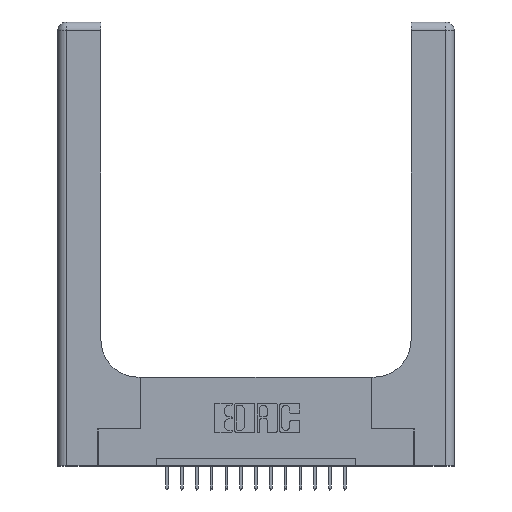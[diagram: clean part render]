
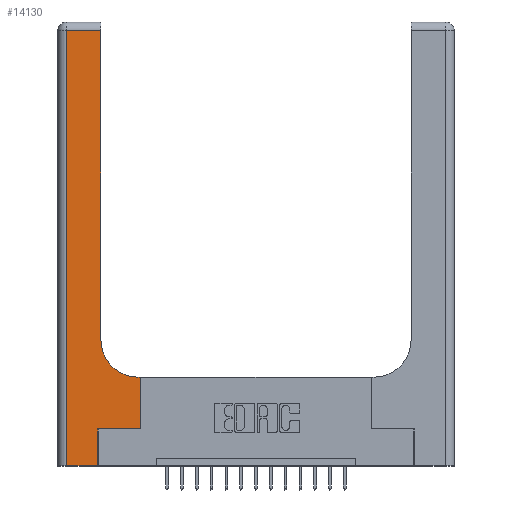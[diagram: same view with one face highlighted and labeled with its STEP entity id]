
A CAD part, top view. The second image highlights one B-rep face of the part: STEP entity #14130.
In plain terms, the highlighted planar face has unit normal (0, 0, 1).
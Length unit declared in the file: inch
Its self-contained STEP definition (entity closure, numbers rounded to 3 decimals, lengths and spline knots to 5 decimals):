
#91 = CARTESIAN_POINT ( 'NONE',  ( 0.2915, 3., 0.37 ) ) ;
#858 = DIRECTION ( 'NONE',  ( 0., 1., 0. ) ) ;
#987 = VECTOR ( 'NONE', #13800, 39.37008 ) ;
#1414 = ORIENTED_EDGE ( 'NONE', *, *, #1818, .T. ) ;
#1717 = CARTESIAN_POINT ( 'NONE',  ( 0.2915, 0.6, 0.37 ) ) ;
#1818 = EDGE_CURVE ( 'NONE', #18265, #15217, #3611, .T. ) ;
#1908 = CARTESIAN_POINT ( 'NONE',  ( 0.06, 0., 0.37 ) ) ;
#2153 = LINE ( 'NONE', #5786, #16778 ) ;
#2196 = ORIENTED_EDGE ( 'NONE', *, *, #6214, .T. ) ;
#2522 = DIRECTION ( 'NONE',  ( 0., 0., -1. ) ) ;
#2661 = DIRECTION ( 'NONE',  ( 1., 0., 0. ) ) ;
#2666 = ORIENTED_EDGE ( 'NONE', *, *, #7473, .T. ) ;
#2772 = VERTEX_POINT ( 'NONE', #1908 ) ;
#2823 = VECTOR ( 'NONE', #11166, 39.37008 ) ;
#3020 = DIRECTION ( 'NONE',  ( 0., 1., 0. ) ) ;
#3329 = VECTOR ( 'NONE', #18202, 39.37008 ) ;
#3611 = CIRCLE ( 'NONE', #15936, 0.25 ) ;
#3687 = ORIENTED_EDGE ( 'NONE', *, *, #12773, .T. ) ;
#4077 = CARTESIAN_POINT ( 'NONE',  ( 0.5415, 0.85, 0.37 ) ) ;
#4161 = EDGE_CURVE ( 'NONE', #15096, #11224, #2153, .T. ) ;
#4436 = ORIENTED_EDGE ( 'NONE', *, *, #16899, .T. ) ;
#4519 = VERTEX_POINT ( 'NONE', #13186 ) ;
#5191 = ORIENTED_EDGE ( 'NONE', *, *, #16734, .T. ) ;
#5257 = CARTESIAN_POINT ( 'NONE',  ( 0.2915, 0.85, 0.37 ) ) ;
#5313 = DIRECTION ( 'NONE',  ( 0., 1., 0. ) ) ;
#5616 = DIRECTION ( 'NONE',  ( -1., 0., 0. ) ) ;
#5687 = CARTESIAN_POINT ( 'NONE',  ( 0., 2.94, 0.37 ) ) ;
#5735 = VECTOR ( 'NONE', #3020, 39.37008 ) ;
#5786 = CARTESIAN_POINT ( 'NONE',  ( 0.5585, 0.25, 0.37 ) ) ;
#6214 = EDGE_CURVE ( 'NONE', #4519, #2772, #14758, .T. ) ;
#6222 = CARTESIAN_POINT ( 'NONE',  ( 0.5585, 0.25, 0.37 ) ) ;
#6415 = VECTOR ( 'NONE', #858, 39.37008 ) ;
#7250 = CARTESIAN_POINT ( 'NONE',  ( 0.5585, 0.6, 0.37 ) ) ;
#7461 = VECTOR ( 'NONE', #5616, 39.37008 ) ;
#7473 = EDGE_CURVE ( 'NONE', #11224, #18265, #11968, .T. ) ;
#7494 = EDGE_LOOP ( 'NONE', ( #3687, #7683, #2196, #4436, #8597, #5191, #10082, #2666, #1414 ) ) ;
#7683 = ORIENTED_EDGE ( 'NONE', *, *, #18147, .T. ) ;
#8170 = PLANE ( 'NONE',  #11395 ) ;
#8458 = VERTEX_POINT ( 'NONE', #8619 ) ;
#8523 = DIRECTION ( 'NONE',  ( 1., 0., 0. ) ) ;
#8597 = ORIENTED_EDGE ( 'NONE', *, *, #13118, .T. ) ;
#8619 = CARTESIAN_POINT ( 'NONE',  ( 0.2915, 2.94, 0.37 ) ) ;
#9448 = CARTESIAN_POINT ( 'NONE',  ( 0.269, 0.25, 0.37 ) ) ;
#9609 = LINE ( 'NONE', #91, #5735 ) ;
#10082 = ORIENTED_EDGE ( 'NONE', *, *, #4161, .T. ) ;
#10148 = LINE ( 'NONE', #11226, #11975 ) ;
#10279 = CARTESIAN_POINT ( 'NONE',  ( 0.5415, 0.6, 0.37 ) ) ;
#10475 = FACE_OUTER_BOUND ( 'NONE', #7494, .T. ) ;
#11166 = DIRECTION ( 'NONE',  ( 1., 0., 0. ) ) ;
#11224 = VERTEX_POINT ( 'NONE', #7250 ) ;
#11226 = CARTESIAN_POINT ( 'NONE',  ( 0., 0., 0.37 ) ) ;
#11395 = AXIS2_PLACEMENT_3D ( 'NONE', #12584, #14064, #15510 ) ;
#11899 = VERTEX_POINT ( 'NONE', #15185 ) ;
#11968 = LINE ( 'NONE', #1717, #987 ) ;
#11975 = VECTOR ( 'NONE', #8523, 39.37008 ) ;
#12584 = CARTESIAN_POINT ( 'NONE',  ( 0., 3., 0.37 ) ) ;
#12773 = EDGE_CURVE ( 'NONE', #15217, #8458, #9609, .T. ) ;
#13118 = EDGE_CURVE ( 'NONE', #11899, #17457, #13498, .T. ) ;
#13186 = CARTESIAN_POINT ( 'NONE',  ( 0.06, 2.94, 0.37 ) ) ;
#13498 = LINE ( 'NONE', #18502, #6415 ) ;
#13800 = DIRECTION ( 'NONE',  ( -1., 0., 0. ) ) ;
#14064 = DIRECTION ( 'NONE',  ( 0., 0., -1. ) ) ;
#14130 = ADVANCED_FACE ( 'NONE', ( #10475 ), #8170, .F. ) ;
#14758 = LINE ( 'NONE', #16720, #3329 ) ;
#15096 = VERTEX_POINT ( 'NONE', #6222 ) ;
#15185 = CARTESIAN_POINT ( 'NONE',  ( 0.269, 0., 0.37 ) ) ;
#15217 = VERTEX_POINT ( 'NONE', #5257 ) ;
#15225 = LINE ( 'NONE', #5687, #7461 ) ;
#15510 = DIRECTION ( 'NONE',  ( -1., 0., 0. ) ) ;
#15852 = CARTESIAN_POINT ( 'NONE',  ( 0.269, 0.25, 0.37 ) ) ;
#15936 = AXIS2_PLACEMENT_3D ( 'NONE', #4077, #2522, #2661 ) ;
#16720 = CARTESIAN_POINT ( 'NONE',  ( 0.06, 3., 0.37 ) ) ;
#16734 = EDGE_CURVE ( 'NONE', #17457, #15096, #17012, .T. ) ;
#16778 = VECTOR ( 'NONE', #5313, 39.37008 ) ;
#16899 = EDGE_CURVE ( 'NONE', #2772, #11899, #10148, .T. ) ;
#17012 = LINE ( 'NONE', #9448, #2823 ) ;
#17457 = VERTEX_POINT ( 'NONE', #15852 ) ;
#18147 = EDGE_CURVE ( 'NONE', #8458, #4519, #15225, .T. ) ;
#18202 = DIRECTION ( 'NONE',  ( 0., -1., 0. ) ) ;
#18265 = VERTEX_POINT ( 'NONE', #10279 ) ;
#18502 = CARTESIAN_POINT ( 'NONE',  ( 0.269, 0., 0.37 ) ) ;
